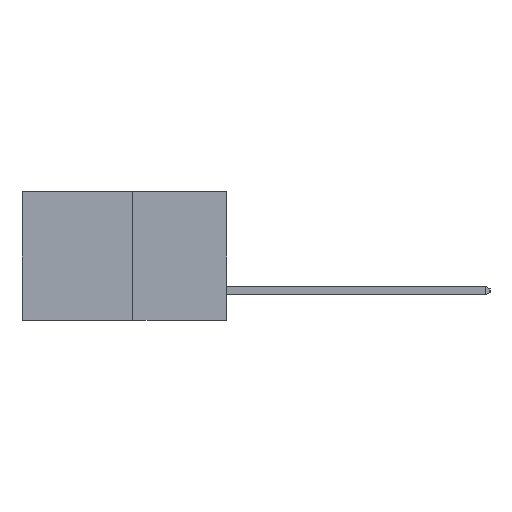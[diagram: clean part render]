
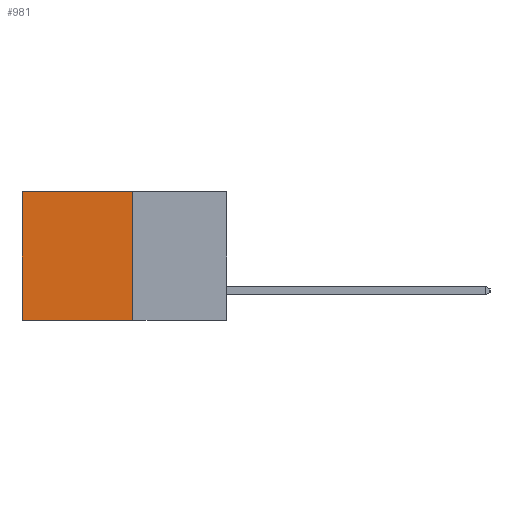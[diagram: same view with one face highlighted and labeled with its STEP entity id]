
A CAD part, left-side view. The second image highlights one B-rep face of the part: STEP entity #981.
In plain terms, the highlighted planar face has unit normal (-1, 0, 0).
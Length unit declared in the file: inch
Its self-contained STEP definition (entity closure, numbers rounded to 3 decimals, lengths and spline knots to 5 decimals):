
#485 = DIRECTION ( 'NONE',  ( 0., 1., 0. ) ) ;
#901 = LINE ( 'NONE', #9327, #5951 ) ;
#981 = ADVANCED_FACE ( 'NONE', ( #9258 ), #6967, .F. ) ;
#1987 = VERTEX_POINT ( 'NONE', #9285 ) ;
#2000 = AXIS2_PLACEMENT_3D ( 'NONE', #6718, #3560, #3652 ) ;
#3166 = CARTESIAN_POINT ( 'NONE',  ( 0.277, 0.27, -0.37 ) ) ;
#3174 = LINE ( 'NONE', #7436, #5821 ) ;
#3560 = DIRECTION ( 'NONE',  ( 1., 0., 0. ) ) ;
#3652 = DIRECTION ( 'NONE',  ( 0., 0., -1. ) ) ;
#3731 = ORIENTED_EDGE ( 'NONE', *, *, #4677, .T. ) ;
#3745 = VECTOR ( 'NONE', #4197, 39.37008 ) ;
#4062 = ORIENTED_EDGE ( 'NONE', *, *, #4982, .F. ) ;
#4197 = DIRECTION ( 'NONE',  ( 0., 1., 0. ) ) ;
#4238 = VECTOR ( 'NONE', #12285, 39.37008 ) ;
#4290 = EDGE_LOOP ( 'NONE', ( #3731, #4062, #9721, #12473 ) ) ;
#4579 = DIRECTION ( 'NONE',  ( 0., 0., -1. ) ) ;
#4677 = EDGE_CURVE ( 'NONE', #12236, #9697, #11780, .T. ) ;
#4982 = EDGE_CURVE ( 'NONE', #7777, #9697, #8867, .T. ) ;
#5821 = VECTOR ( 'NONE', #485, 39.37008 ) ;
#5951 = VECTOR ( 'NONE', #4579, 39.37008 ) ;
#6032 = CARTESIAN_POINT ( 'NONE',  ( 0.277, 0.59, 0. ) ) ;
#6718 = CARTESIAN_POINT ( 'NONE',  ( 0.277, 0.27, -0.37 ) ) ;
#6967 = PLANE ( 'NONE',  #2000 ) ;
#7436 = CARTESIAN_POINT ( 'NONE',  ( 0.277, 0.27, 0. ) ) ;
#7777 = VERTEX_POINT ( 'NONE', #9531 ) ;
#8867 = LINE ( 'NONE', #3166, #3745 ) ;
#9258 = FACE_OUTER_BOUND ( 'NONE', #4290, .T. ) ;
#9285 = CARTESIAN_POINT ( 'NONE',  ( 0.277, 0.27, 0. ) ) ;
#9327 = CARTESIAN_POINT ( 'NONE',  ( 0.277, 0.27, -0.37 ) ) ;
#9500 = EDGE_CURVE ( 'NONE', #1987, #12236, #3174, .T. ) ;
#9531 = CARTESIAN_POINT ( 'NONE',  ( 0.277, 0.27, -0.37 ) ) ;
#9697 = VERTEX_POINT ( 'NONE', #11402 ) ;
#9721 = ORIENTED_EDGE ( 'NONE', *, *, #10100, .F. ) ;
#10100 = EDGE_CURVE ( 'NONE', #1987, #7777, #901, .T. ) ;
#11358 = CARTESIAN_POINT ( 'NONE',  ( 0.277, 0.59, -0.37 ) ) ;
#11402 = CARTESIAN_POINT ( 'NONE',  ( 0.277, 0.59, -0.37 ) ) ;
#11780 = LINE ( 'NONE', #11358, #4238 ) ;
#12236 = VERTEX_POINT ( 'NONE', #6032 ) ;
#12285 = DIRECTION ( 'NONE',  ( 0., 0., -1. ) ) ;
#12473 = ORIENTED_EDGE ( 'NONE', *, *, #9500, .T. ) ;
